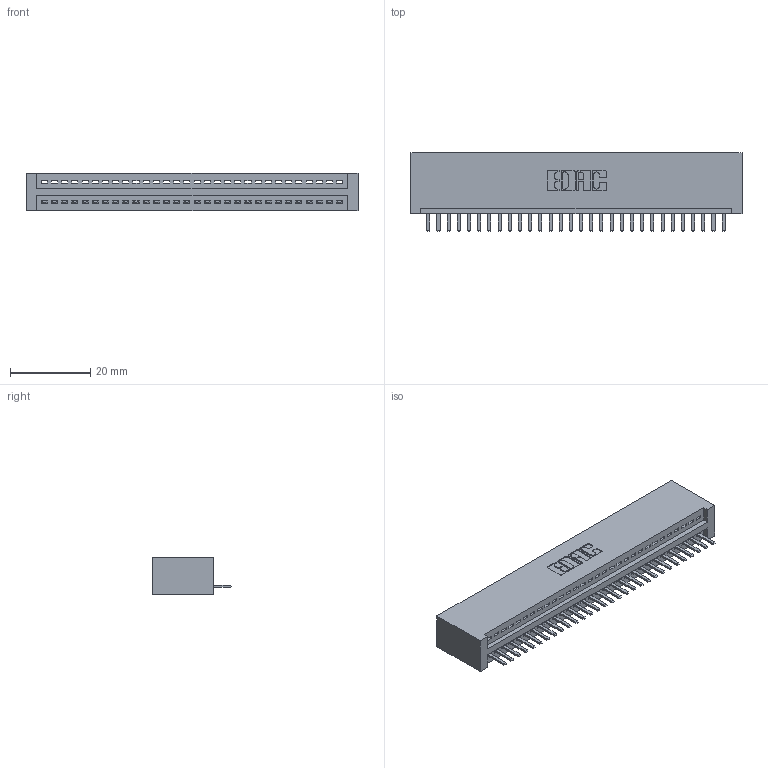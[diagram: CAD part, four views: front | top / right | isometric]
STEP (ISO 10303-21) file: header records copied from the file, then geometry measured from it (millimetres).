
FILE_DESCRIPTION (( 'STEP AP203' ), '1' );
FILE_NAME ('395-030-520-101.STEP', '2018-11-10T22:19:02', ( '' ), ( '' ), 'SwSTEP 2.0', 'SolidWorks 2016', '' );
FILE_SCHEMA (( 'CONFIG_CONTROL_DESIGN' ));
Length unit declared in the file: inch
Products named in the file (3): 345 Part_No Mounting Lugs; 395-030-520-101; 345-292-001_345-293-120
Assembly tree (31 placements, depth 2):
  395-030-520-101
    345 Part_No Mounting Lugs
    345-292-001_345-293-120  x30
Bounding box: 82.8 x 19.68 x 9.4 mm (x, y, z)
Volume: 8264.6 mm3; surface area: 10727.6 mm2
Topology: 31 solids, 31 shells, 1978 faces, 5837 edges, 3810 vertices
Faces by surface type: plane 1336, cylinder 642
Entity records: 24031 total; most frequent: CARTESIAN_POINT 4182, ORIENTED_EDGE 4134, DIRECTION 3651, EDGE_CURVE 2067, VECTOR 1819, LINE 1819, VERTEX_POINT 1374, AXIS2_PLACEMENT_3D 916
